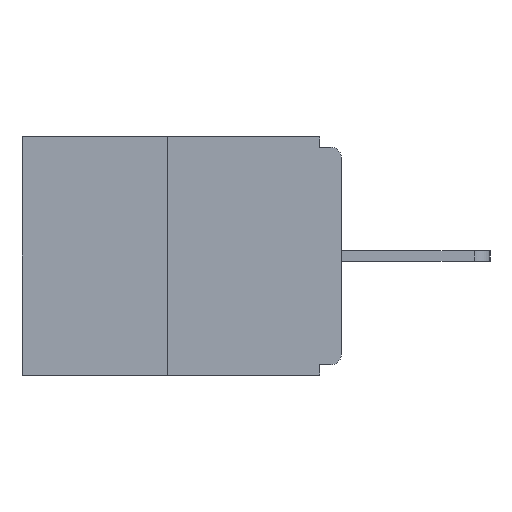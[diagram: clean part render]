
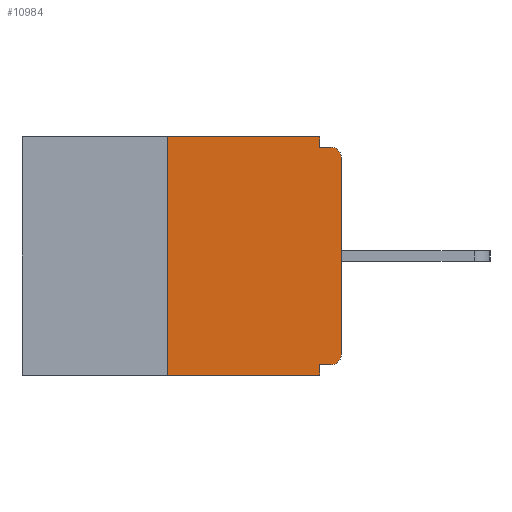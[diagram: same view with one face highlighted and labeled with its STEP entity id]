
A CAD part, left-side view. The second image highlights one B-rep face of the part: STEP entity #10984.
In plain terms, the highlighted planar face has unit normal (-1, 0, 0).
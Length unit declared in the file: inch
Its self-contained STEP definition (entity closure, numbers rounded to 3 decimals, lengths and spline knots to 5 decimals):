
#332 = CARTESIAN_POINT ( 'NONE',  ( 0., 0.031, -0.343 ) ) ;
#380 = AXIS2_PLACEMENT_3D ( 'NONE', #11173, #2013, #10779 ) ;
#413 = ORIENTED_EDGE ( 'NONE', *, *, #11969, .T. ) ;
#485 = CARTESIAN_POINT ( 'NONE',  ( 0., 0.015, -0.03 ) ) ;
#920 = ORIENTED_EDGE ( 'NONE', *, *, #9954, .F. ) ;
#1178 = VERTEX_POINT ( 'NONE', #13137 ) ;
#1706 = DIRECTION ( 'NONE',  ( 0., 0., -1. ) ) ;
#1941 = FACE_OUTER_BOUND ( 'NONE', #10361, .T. ) ;
#2013 = DIRECTION ( 'NONE',  ( 1., 0., 0. ) ) ;
#2206 = VERTEX_POINT ( 'NONE', #4717 ) ;
#2340 = LINE ( 'NONE', #15556, #13183 ) ;
#2499 = VECTOR ( 'NONE', #1706, 39.37008 ) ;
#2602 = CARTESIAN_POINT ( 'NONE',  ( 0., 0.031, -0.343 ) ) ;
#2673 = EDGE_CURVE ( 'NONE', #17637, #1178, #9807, .T. ) ;
#2873 = VECTOR ( 'NONE', #15388, 39.37008 ) ;
#3139 = CARTESIAN_POINT ( 'NONE',  ( 0., 0.25, 0. ) ) ;
#3362 = VECTOR ( 'NONE', #12655, 39.37008 ) ;
#3484 = DIRECTION ( 'NONE',  ( 0., 1., 0. ) ) ;
#3532 = VERTEX_POINT ( 'NONE', #13000 ) ;
#3932 = VECTOR ( 'NONE', #3484, 39.37008 ) ;
#4215 = VECTOR ( 'NONE', #10240, 39.37008 ) ;
#4240 = EDGE_CURVE ( 'NONE', #3532, #2206, #11877, .T. ) ;
#4312 = DIRECTION ( 'NONE',  ( 0., -1., 0. ) ) ;
#4433 = VECTOR ( 'NONE', #16500, 39.37008 ) ;
#4717 = CARTESIAN_POINT ( 'NONE',  ( 0., 0.031, -0.328 ) ) ;
#5196 = AXIS2_PLACEMENT_3D ( 'NONE', #17510, #17578, #16086 ) ;
#5547 = ORIENTED_EDGE ( 'NONE', *, *, #9260, .F. ) ;
#5729 = VERTEX_POINT ( 'NONE', #332 ) ;
#6000 = CARTESIAN_POINT ( 'NONE',  ( 0., 0.031, 0. ) ) ;
#6389 = VECTOR ( 'NONE', #12879, 39.37008 ) ;
#6443 = LINE ( 'NONE', #3139, #4215 ) ;
#6468 = PLANE ( 'NONE',  #380 ) ;
#6654 = CIRCLE ( 'NONE', #5196, 0.015 ) ;
#7109 = CARTESIAN_POINT ( 'NONE',  ( 0., 0., -0.015 ) ) ;
#7199 = VERTEX_POINT ( 'NONE', #10184 ) ;
#7216 = ORIENTED_EDGE ( 'NONE', *, *, #2673, .F. ) ;
#7928 = VERTEX_POINT ( 'NONE', #17834 ) ;
#7981 = ORIENTED_EDGE ( 'NONE', *, *, #17453, .F. ) ;
#8083 = EDGE_CURVE ( 'NONE', #3532, #14105, #6654, .T. ) ;
#8244 = EDGE_CURVE ( 'NONE', #14105, #13207, #11924, .T. ) ;
#8992 = ORIENTED_EDGE ( 'NONE', *, *, #8244, .T. ) ;
#8995 = CARTESIAN_POINT ( 'NONE',  ( 0., 0., -0.03 ) ) ;
#9113 = CARTESIAN_POINT ( 'NONE',  ( 0., 0., -0.328 ) ) ;
#9260 = EDGE_CURVE ( 'NONE', #1178, #7928, #14531, .T. ) ;
#9597 = CIRCLE ( 'NONE', #12230, 0.015 ) ;
#9807 = LINE ( 'NONE', #6000, #2499 ) ;
#9954 = EDGE_CURVE ( 'NONE', #7199, #17637, #10172, .T. ) ;
#10004 = EDGE_CURVE ( 'NONE', #17394, #7199, #6443, .T. ) ;
#10172 = LINE ( 'NONE', #16742, #2873 ) ;
#10184 = CARTESIAN_POINT ( 'NONE',  ( 0., 0.25, 0. ) ) ;
#10240 = DIRECTION ( 'NONE',  ( 0., 0., 1. ) ) ;
#10361 = EDGE_LOOP ( 'NONE', ( #920, #15616, #413, #7981, #10991, #15634, #8992, #15052, #5547, #7216 ) ) ;
#10779 = DIRECTION ( 'NONE',  ( 0., 0., -1. ) ) ;
#10984 = ADVANCED_FACE ( 'NONE', ( #1941 ), #6468, .F. ) ;
#10991 = ORIENTED_EDGE ( 'NONE', *, *, #4240, .F. ) ;
#11173 = CARTESIAN_POINT ( 'NONE',  ( 0., 0.46, 0. ) ) ;
#11499 = CARTESIAN_POINT ( 'NONE',  ( 0., 0.031, 0. ) ) ;
#11668 = DIRECTION ( 'NONE',  ( 0., 0., -1. ) ) ;
#11877 = LINE ( 'NONE', #9113, #3932 ) ;
#11924 = LINE ( 'NONE', #12168, #4433 ) ;
#11969 = EDGE_CURVE ( 'NONE', #17394, #5729, #2340, .T. ) ;
#12168 = CARTESIAN_POINT ( 'NONE',  ( 0., 0., 0. ) ) ;
#12230 = AXIS2_PLACEMENT_3D ( 'NONE', #485, #17205, #11668 ) ;
#12422 = LINE ( 'NONE', #2602, #3362 ) ;
#12655 = DIRECTION ( 'NONE',  ( 0., 0., -1. ) ) ;
#12879 = DIRECTION ( 'NONE',  ( 0., -1., 0. ) ) ;
#13000 = CARTESIAN_POINT ( 'NONE',  ( 0., 0.015, -0.328 ) ) ;
#13137 = CARTESIAN_POINT ( 'NONE',  ( 0., 0.031, -0.015 ) ) ;
#13183 = VECTOR ( 'NONE', #4312, 39.37008 ) ;
#13207 = VERTEX_POINT ( 'NONE', #8995 ) ;
#14105 = VERTEX_POINT ( 'NONE', #14827 ) ;
#14390 = EDGE_CURVE ( 'NONE', #13207, #7928, #9597, .T. ) ;
#14531 = LINE ( 'NONE', #7109, #6389 ) ;
#14827 = CARTESIAN_POINT ( 'NONE',  ( 0., 0., -0.313 ) ) ;
#15052 = ORIENTED_EDGE ( 'NONE', *, *, #14390, .T. ) ;
#15388 = DIRECTION ( 'NONE',  ( 0., -1., 0. ) ) ;
#15556 = CARTESIAN_POINT ( 'NONE',  ( 0., 0.46, -0.343 ) ) ;
#15616 = ORIENTED_EDGE ( 'NONE', *, *, #10004, .F. ) ;
#15634 = ORIENTED_EDGE ( 'NONE', *, *, #8083, .T. ) ;
#16086 = DIRECTION ( 'NONE',  ( 0., 0., -1. ) ) ;
#16500 = DIRECTION ( 'NONE',  ( 0., 0., 1. ) ) ;
#16742 = CARTESIAN_POINT ( 'NONE',  ( 0., 0.46, 0. ) ) ;
#17108 = CARTESIAN_POINT ( 'NONE',  ( 0., 0.25, -0.343 ) ) ;
#17205 = DIRECTION ( 'NONE',  ( -1., 0., 0. ) ) ;
#17394 = VERTEX_POINT ( 'NONE', #17108 ) ;
#17453 = EDGE_CURVE ( 'NONE', #2206, #5729, #12422, .T. ) ;
#17510 = CARTESIAN_POINT ( 'NONE',  ( 0., 0.015, -0.313 ) ) ;
#17578 = DIRECTION ( 'NONE',  ( -1., 0., 0. ) ) ;
#17637 = VERTEX_POINT ( 'NONE', #11499 ) ;
#17834 = CARTESIAN_POINT ( 'NONE',  ( 0., 0.015, -0.015 ) ) ;
